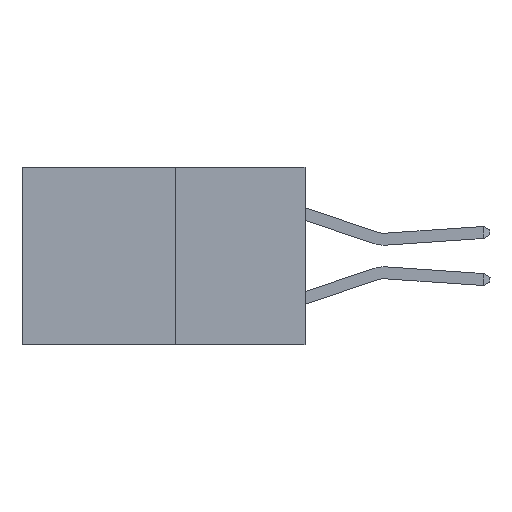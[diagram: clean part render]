
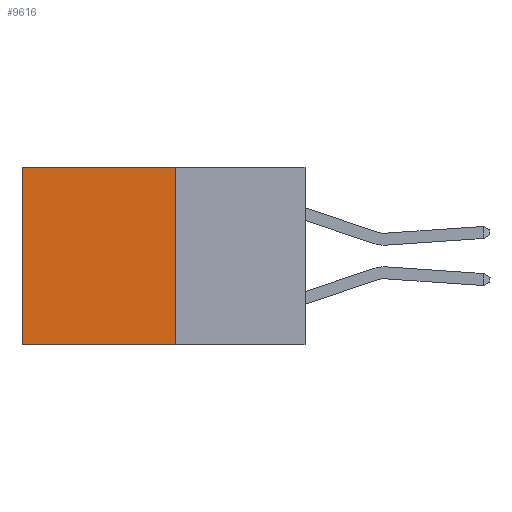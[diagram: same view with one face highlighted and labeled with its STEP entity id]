
A CAD part, left-side view. The second image highlights one B-rep face of the part: STEP entity #9616.
In plain terms, the highlighted planar face has unit normal (-1, 0, 0).
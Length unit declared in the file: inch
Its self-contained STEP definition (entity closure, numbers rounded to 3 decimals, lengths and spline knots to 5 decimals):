
#1186 = VERTEX_POINT ( 'NONE', #12298 ) ;
#3212 = VERTEX_POINT ( 'NONE', #13188 ) ;
#3777 = ORIENTED_EDGE ( 'NONE', *, *, #10282, .F. ) ;
#4792 = AXIS2_PLACEMENT_3D ( 'NONE', #5410, #17301, #7140 ) ;
#4836 = CARTESIAN_POINT ( 'NONE',  ( 0.277, 0.59, -0.37 ) ) ;
#5410 = CARTESIAN_POINT ( 'NONE',  ( 0.277, 0.27, -0.37 ) ) ;
#5595 = ORIENTED_EDGE ( 'NONE', *, *, #14092, .T. ) ;
#6576 = CARTESIAN_POINT ( 'NONE',  ( 0.277, 0.27, -0.37 ) ) ;
#7140 = DIRECTION ( 'NONE',  ( 0., 0., -1. ) ) ;
#7978 = ORIENTED_EDGE ( 'NONE', *, *, #21585, .F. ) ;
#8667 = DIRECTION ( 'NONE',  ( 0., 1., 0. ) ) ;
#9616 = ADVANCED_FACE ( 'NONE', ( #20770 ), #20619, .F. ) ;
#10282 = EDGE_CURVE ( 'NONE', #3212, #12230, #11877, .T. ) ;
#11877 = LINE ( 'NONE', #18835, #12393 ) ;
#12230 = VERTEX_POINT ( 'NONE', #21946 ) ;
#12247 = VECTOR ( 'NONE', #13303, 39.37008 ) ;
#12298 = CARTESIAN_POINT ( 'NONE',  ( 0.277, 0.59, 0. ) ) ;
#12393 = VECTOR ( 'NONE', #8667, 39.37008 ) ;
#12525 = CARTESIAN_POINT ( 'NONE',  ( 0.277, 0.27, 0. ) ) ;
#12931 = VECTOR ( 'NONE', #13315, 39.37008 ) ;
#13054 = CARTESIAN_POINT ( 'NONE',  ( 0.277, 0.27, 0. ) ) ;
#13188 = CARTESIAN_POINT ( 'NONE',  ( 0.277, 0.27, -0.37 ) ) ;
#13303 = DIRECTION ( 'NONE',  ( 0., 0., -1. ) ) ;
#13315 = DIRECTION ( 'NONE',  ( 0., 0., -1. ) ) ;
#14092 = EDGE_CURVE ( 'NONE', #1186, #12230, #17326, .T. ) ;
#14693 = LINE ( 'NONE', #13054, #18169 ) ;
#16402 = DIRECTION ( 'NONE',  ( 0., 1., 0. ) ) ;
#17269 = EDGE_CURVE ( 'NONE', #21863, #1186, #14693, .T. ) ;
#17301 = DIRECTION ( 'NONE',  ( 1., 0., 0. ) ) ;
#17326 = LINE ( 'NONE', #4836, #12247 ) ;
#17384 = ORIENTED_EDGE ( 'NONE', *, *, #17269, .T. ) ;
#18169 = VECTOR ( 'NONE', #16402, 39.37008 ) ;
#18613 = EDGE_LOOP ( 'NONE', ( #5595, #3777, #7978, #17384 ) ) ;
#18835 = CARTESIAN_POINT ( 'NONE',  ( 0.277, 0.27, -0.37 ) ) ;
#20619 = PLANE ( 'NONE',  #4792 ) ;
#20770 = FACE_OUTER_BOUND ( 'NONE', #18613, .T. ) ;
#21426 = LINE ( 'NONE', #6576, #12931 ) ;
#21585 = EDGE_CURVE ( 'NONE', #21863, #3212, #21426, .T. ) ;
#21863 = VERTEX_POINT ( 'NONE', #12525 ) ;
#21946 = CARTESIAN_POINT ( 'NONE',  ( 0.277, 0.59, -0.37 ) ) ;
